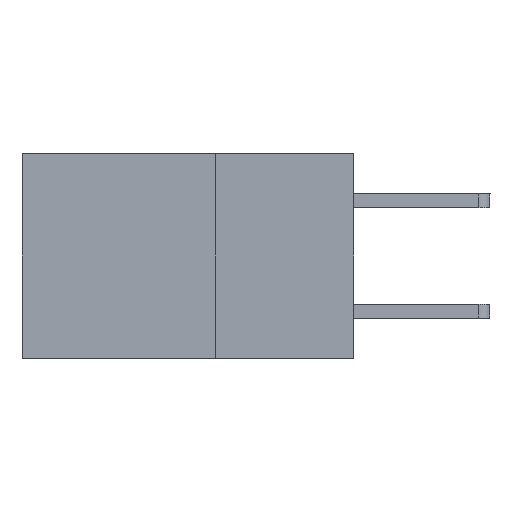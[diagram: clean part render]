
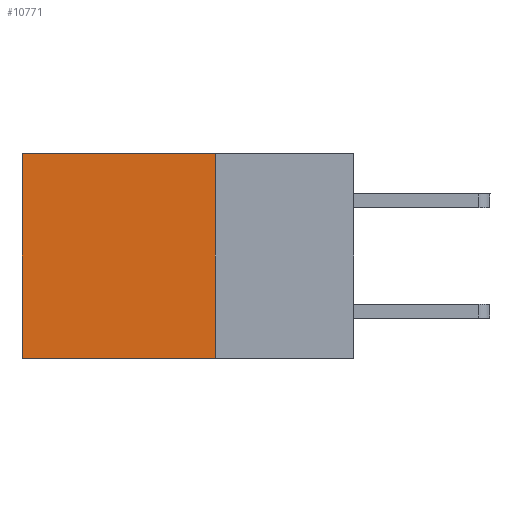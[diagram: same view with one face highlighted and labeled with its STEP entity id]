
A CAD part, left-side view. The second image highlights one B-rep face of the part: STEP entity #10771.
In plain terms, the highlighted planar face has unit normal (-1, 0, 0).
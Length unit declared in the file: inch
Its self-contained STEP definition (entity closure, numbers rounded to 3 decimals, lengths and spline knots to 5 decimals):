
#46 = CARTESIAN_POINT ( 'NONE',  ( 0.2875, 0.25, 0. ) ) ;
#636 = DIRECTION ( 'NONE',  ( 0., 0., -1. ) ) ;
#943 = CARTESIAN_POINT ( 'NONE',  ( 0.2875, 0.6, -0.37 ) ) ;
#1189 = VECTOR ( 'NONE', #3508, 39.37008 ) ;
#1986 = VECTOR ( 'NONE', #7216, 39.37008 ) ;
#2272 = EDGE_LOOP ( 'NONE', ( #11599, #11040, #4135, #5994 ) ) ;
#3051 = VECTOR ( 'NONE', #6487, 39.37008 ) ;
#3508 = DIRECTION ( 'NONE',  ( 0., 1., 0. ) ) ;
#4135 = ORIENTED_EDGE ( 'NONE', *, *, #8032, .F. ) ;
#4351 = LINE ( 'NONE', #12442, #9333 ) ;
#4506 = CARTESIAN_POINT ( 'NONE',  ( 0.2875, 0.25, -0.37 ) ) ;
#4781 = VERTEX_POINT ( 'NONE', #5841 ) ;
#4906 = VERTEX_POINT ( 'NONE', #943 ) ;
#5036 = PLANE ( 'NONE',  #6296 ) ;
#5470 = EDGE_CURVE ( 'NONE', #9057, #4781, #11108, .T. ) ;
#5626 = EDGE_CURVE ( 'NONE', #6481, #4906, #6650, .T. ) ;
#5841 = CARTESIAN_POINT ( 'NONE',  ( 0.2875, 0.6, 0. ) ) ;
#5994 = ORIENTED_EDGE ( 'NONE', *, *, #5470, .T. ) ;
#6079 = DIRECTION ( 'NONE',  ( 0., 0., -1. ) ) ;
#6296 = AXIS2_PLACEMENT_3D ( 'NONE', #9917, #11771, #6079 ) ;
#6481 = VERTEX_POINT ( 'NONE', #7450 ) ;
#6487 = DIRECTION ( 'NONE',  ( 0., 0., -1. ) ) ;
#6650 = LINE ( 'NONE', #4506, #1189 ) ;
#7124 = EDGE_CURVE ( 'NONE', #4781, #4906, #4351, .T. ) ;
#7216 = DIRECTION ( 'NONE',  ( 0., 1., 0. ) ) ;
#7450 = CARTESIAN_POINT ( 'NONE',  ( 0.2875, 0.25, -0.37 ) ) ;
#8032 = EDGE_CURVE ( 'NONE', #9057, #6481, #10906, .T. ) ;
#8063 = CARTESIAN_POINT ( 'NONE',  ( 0.2875, 0.25, 0. ) ) ;
#8398 = CARTESIAN_POINT ( 'NONE',  ( 0.2875, 0.25, 0. ) ) ;
#9057 = VERTEX_POINT ( 'NONE', #46 ) ;
#9333 = VECTOR ( 'NONE', #636, 39.37008 ) ;
#9917 = CARTESIAN_POINT ( 'NONE',  ( 0.2875, 0.25, 0. ) ) ;
#10124 = FACE_OUTER_BOUND ( 'NONE', #2272, .T. ) ;
#10771 = ADVANCED_FACE ( 'NONE', ( #10124 ), #5036, .F. ) ;
#10906 = LINE ( 'NONE', #8398, #3051 ) ;
#11040 = ORIENTED_EDGE ( 'NONE', *, *, #5626, .F. ) ;
#11108 = LINE ( 'NONE', #8063, #1986 ) ;
#11599 = ORIENTED_EDGE ( 'NONE', *, *, #7124, .T. ) ;
#11771 = DIRECTION ( 'NONE',  ( 1., 0., 0. ) ) ;
#12442 = CARTESIAN_POINT ( 'NONE',  ( 0.2875, 0.6, 0. ) ) ;
